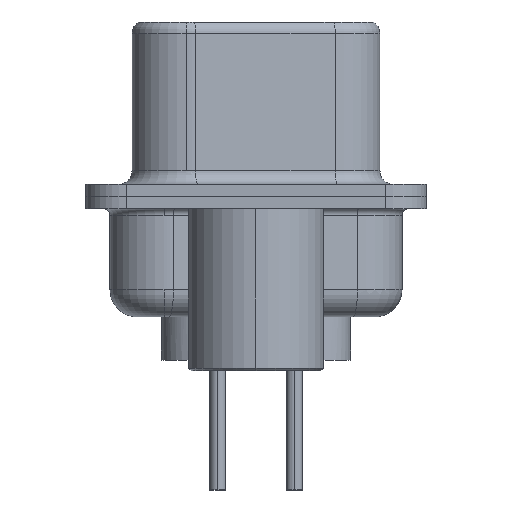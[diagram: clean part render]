
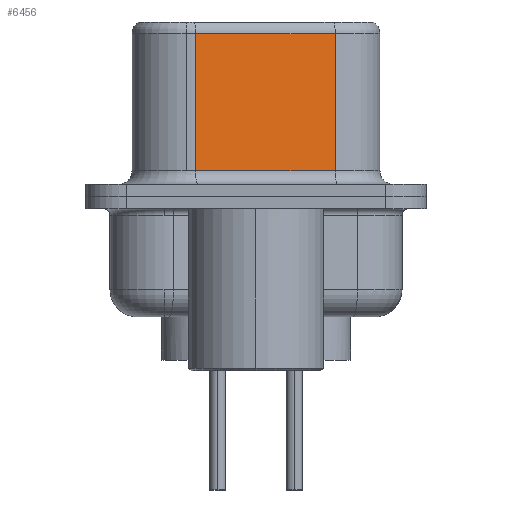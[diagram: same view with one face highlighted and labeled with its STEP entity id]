
A CAD part, left-side view. The second image highlights one B-rep face of the part: STEP entity #6456.
In plain terms, the highlighted planar face has unit normal (-0.985, -0.174, 0).
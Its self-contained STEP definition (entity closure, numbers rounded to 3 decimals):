
#1857 = CARTESIAN_POINT ( 'NONE',  ( 4.575, -2.927, 0.95 ) ) ;
#3876 = PLANE ( 'NONE',  #9687 ) ;
#3953 = CARTESIAN_POINT ( 'NONE',  ( 4.575, -2.927, 6.02 ) ) ;
#4003 = EDGE_LOOP ( 'NONE', ( #8699, #15759, #16768, #6863 ) ) ;
#4083 = CARTESIAN_POINT ( 'NONE',  ( 3.665, 2.233, 0.95 ) ) ;
#4205 = CARTESIAN_POINT ( 'NONE',  ( 3.665, 2.233, 6.02 ) ) ;
#4228 = DIRECTION ( 'NONE',  ( -0.174, 0.985, 0. ) ) ;
#4427 = CARTESIAN_POINT ( 'NONE',  ( 4.575, -2.927, 6.02 ) ) ;
#4784 = EDGE_CURVE ( 'NONE', #9270, #13576, #5362, .T. ) ;
#5207 = VERTEX_POINT ( 'NONE', #4427 ) ;
#5362 = LINE ( 'NONE', #17003, #17703 ) ;
#6456 = ADVANCED_FACE ( 'NONE', ( #11273 ), #3876, .F. ) ;
#6759 = EDGE_CURVE ( 'NONE', #13576, #10992, #13565, .T. ) ;
#6832 = DIRECTION ( 'NONE',  ( 0., 0., -1. ) ) ;
#6863 = ORIENTED_EDGE ( 'NONE', *, *, #6759, .T. ) ;
#7072 = CARTESIAN_POINT ( 'NONE',  ( 4.575, -2.927, 6.52 ) ) ;
#7807 = VECTOR ( 'NONE', #6832, 1000. ) ;
#7914 = LINE ( 'NONE', #13928, #7807 ) ;
#8692 = VECTOR ( 'NONE', #4228, 1000. ) ;
#8699 = ORIENTED_EDGE ( 'NONE', *, *, #13410, .F. ) ;
#9270 = VERTEX_POINT ( 'NONE', #4205 ) ;
#9687 = AXIS2_PLACEMENT_3D ( 'NONE', #7072, #9809, #15722 ) ;
#9809 = DIRECTION ( 'NONE',  ( 0.985, 0.174, 0. ) ) ;
#10651 = CARTESIAN_POINT ( 'NONE',  ( 4.575, -2.927, 0.95 ) ) ;
#10992 = VERTEX_POINT ( 'NONE', #1857 ) ;
#11273 = FACE_OUTER_BOUND ( 'NONE', #4003, .T. ) ;
#11514 = EDGE_CURVE ( 'NONE', #5207, #9270, #17331, .T. ) ;
#13410 = EDGE_CURVE ( 'NONE', #5207, #10992, #7914, .T. ) ;
#13565 = LINE ( 'NONE', #10651, #14343 ) ;
#13576 = VERTEX_POINT ( 'NONE', #4083 ) ;
#13928 = CARTESIAN_POINT ( 'NONE',  ( 4.575, -2.927, 6.52 ) ) ;
#14343 = VECTOR ( 'NONE', #18215, 1000. ) ;
#15376 = DIRECTION ( 'NONE',  ( 0., 0., -1. ) ) ;
#15722 = DIRECTION ( 'NONE',  ( -0.174, 0.985, 0. ) ) ;
#15759 = ORIENTED_EDGE ( 'NONE', *, *, #11514, .T. ) ;
#16768 = ORIENTED_EDGE ( 'NONE', *, *, #4784, .T. ) ;
#17003 = CARTESIAN_POINT ( 'NONE',  ( 3.665, 2.233, 6.52 ) ) ;
#17331 = LINE ( 'NONE', #3953, #8692 ) ;
#17703 = VECTOR ( 'NONE', #15376, 1000. ) ;
#18215 = DIRECTION ( 'NONE',  ( 0.174, -0.985, 0. ) ) ;
